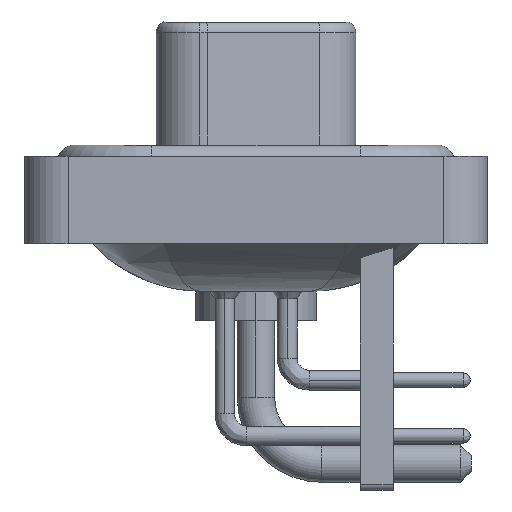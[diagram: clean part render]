
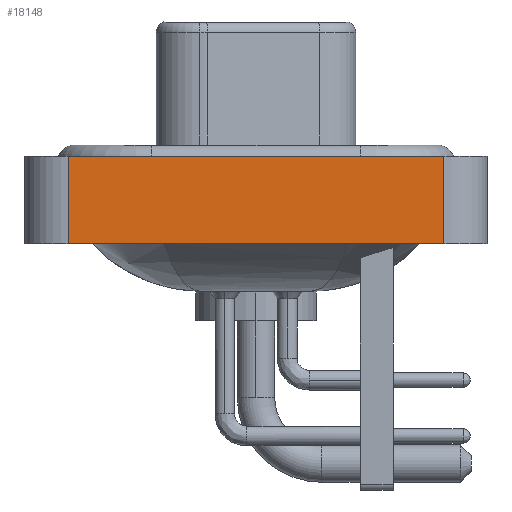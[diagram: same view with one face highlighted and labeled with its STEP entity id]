
A CAD part, left-side view. The second image highlights one B-rep face of the part: STEP entity #18148.
In plain terms, the highlighted planar face has unit normal (-1, 0, 0).
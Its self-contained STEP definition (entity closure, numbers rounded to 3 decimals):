
#718 = LINE ( 'NONE', #19386, #15577 ) ;
#1734 = AXIS2_PLACEMENT_3D ( 'NONE', #8405, #6101, #18282 ) ;
#2721 = EDGE_CURVE ( 'NONE', #20869, #8068, #21747, .T. ) ;
#3266 = VECTOR ( 'NONE', #19854, 1000. ) ;
#3915 = VERTEX_POINT ( 'NONE', #22339 ) ;
#4104 = EDGE_LOOP ( 'NONE', ( #22174, #22424, #25673, #18449 ) ) ;
#4646 = EDGE_CURVE ( 'NONE', #22707, #3915, #5118, .T. ) ;
#4849 = DIRECTION ( 'NONE',  ( 0., 0., 1. ) ) ;
#5118 = LINE ( 'NONE', #11592, #10252 ) ;
#6101 = DIRECTION ( 'NONE',  ( -1., 0., 0. ) ) ;
#6237 = PLANE ( 'NONE',  #1734 ) ;
#6529 = DIRECTION ( 'NONE',  ( 0., -1., 0. ) ) ;
#7653 = CARTESIAN_POINT ( 'NONE',  ( -7.3, -8.55, -3.6 ) ) ;
#8068 = VERTEX_POINT ( 'NONE', #24108 ) ;
#8405 = CARTESIAN_POINT ( 'NONE',  ( -7.3, -8.55, -3.6 ) ) ;
#10031 = FACE_OUTER_BOUND ( 'NONE', #4104, .T. ) ;
#10252 = VECTOR ( 'NONE', #4849, 1000. ) ;
#11436 = EDGE_CURVE ( 'NONE', #3915, #8068, #718, .T. ) ;
#11592 = CARTESIAN_POINT ( 'NONE',  ( -7.3, 8.55, -3.6 ) ) ;
#12242 = CARTESIAN_POINT ( 'NONE',  ( -7.3, 8.55, -3.6 ) ) ;
#13753 = CARTESIAN_POINT ( 'NONE',  ( -7.3, -8.55, -3.6 ) ) ;
#15577 = VECTOR ( 'NONE', #6529, 1000. ) ;
#15711 = LINE ( 'NONE', #26282, #25080 ) ;
#18126 = EDGE_CURVE ( 'NONE', #22707, #20869, #15711, .T. ) ;
#18148 = ADVANCED_FACE ( 'NONE', ( #10031 ), #6237, .T. ) ;
#18282 = DIRECTION ( 'NONE',  ( 0., 0., 1. ) ) ;
#18449 = ORIENTED_EDGE ( 'NONE', *, *, #18126, .T. ) ;
#19386 = CARTESIAN_POINT ( 'NONE',  ( -7.3, -8.55, 0.4 ) ) ;
#19854 = DIRECTION ( 'NONE',  ( 0., 0., 1. ) ) ;
#20869 = VERTEX_POINT ( 'NONE', #13753 ) ;
#21747 = LINE ( 'NONE', #7653, #3266 ) ;
#22174 = ORIENTED_EDGE ( 'NONE', *, *, #2721, .T. ) ;
#22339 = CARTESIAN_POINT ( 'NONE',  ( -7.3, 8.55, 0.4 ) ) ;
#22424 = ORIENTED_EDGE ( 'NONE', *, *, #11436, .F. ) ;
#22707 = VERTEX_POINT ( 'NONE', #12242 ) ;
#23990 = DIRECTION ( 'NONE',  ( 0., -1., 0. ) ) ;
#24108 = CARTESIAN_POINT ( 'NONE',  ( -7.3, -8.55, 0.4 ) ) ;
#25080 = VECTOR ( 'NONE', #23990, 1000. ) ;
#25673 = ORIENTED_EDGE ( 'NONE', *, *, #4646, .F. ) ;
#26282 = CARTESIAN_POINT ( 'NONE',  ( -7.3, -8.55, -3.6 ) ) ;
